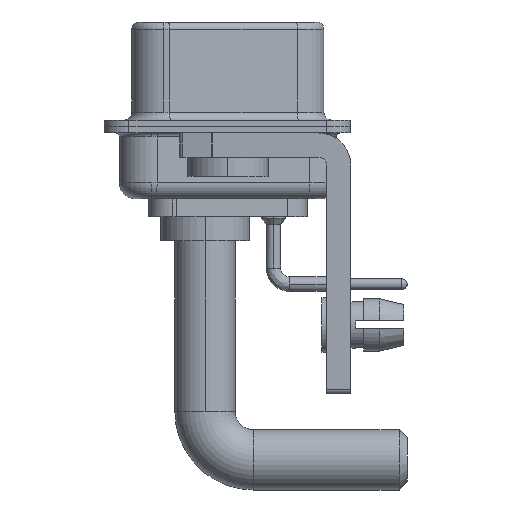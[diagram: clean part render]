
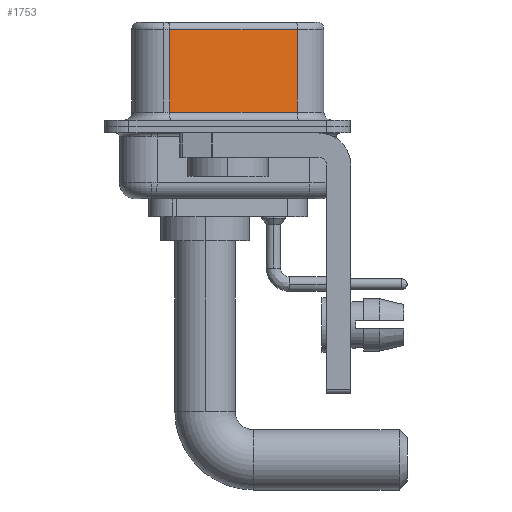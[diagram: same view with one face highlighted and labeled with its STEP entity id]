
A CAD part, left-side view. The second image highlights one B-rep face of the part: STEP entity #1753.
In plain terms, the highlighted planar face has unit normal (-0.985, -0.174, 0).
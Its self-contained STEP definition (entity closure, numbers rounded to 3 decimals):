
#435 = ORIENTED_EDGE ( 'NONE', *, *, #20019, .F. ) ;
#1753 = ADVANCED_FACE ( 'NONE', ( #7805 ), #26014, .F. ) ;
#2427 = LINE ( 'NONE', #4057, #3709 ) ;
#3034 = EDGE_CURVE ( 'NONE', #8544, #25024, #25427, .T. ) ;
#3056 = CARTESIAN_POINT ( 'NONE',  ( 5.132, -4.322, 6.02 ) ) ;
#3384 = CARTESIAN_POINT ( 'NONE',  ( 5.132, -4.322, 6.52 ) ) ;
#3709 = VECTOR ( 'NONE', #14762, 1000. ) ;
#4057 = CARTESIAN_POINT ( 'NONE',  ( 5.132, -4.322, 0.9 ) ) ;
#5459 = DIRECTION ( 'NONE',  ( -0.174, 0.985, 0. ) ) ;
#5599 = DIRECTION ( 'NONE',  ( 0., 0., -1. ) ) ;
#6811 = AXIS2_PLACEMENT_3D ( 'NONE', #3384, #19721, #7542 ) ;
#7191 = EDGE_LOOP ( 'NONE', ( #435, #9378, #7311, #12192 ) ) ;
#7311 = ORIENTED_EDGE ( 'NONE', *, *, #17206, .T. ) ;
#7542 = DIRECTION ( 'NONE',  ( -0.174, 0.985, 0. ) ) ;
#7805 = FACE_OUTER_BOUND ( 'NONE', #7191, .T. ) ;
#8544 = VERTEX_POINT ( 'NONE', #24185 ) ;
#9378 = ORIENTED_EDGE ( 'NONE', *, *, #3034, .T. ) ;
#12192 = ORIENTED_EDGE ( 'NONE', *, *, #13444, .T. ) ;
#13444 = EDGE_CURVE ( 'NONE', #19548, #16206, #2427, .T. ) ;
#14762 = DIRECTION ( 'NONE',  ( 0.174, -0.985, 0. ) ) ;
#15463 = VECTOR ( 'NONE', #21541, 1000. ) ;
#16206 = VERTEX_POINT ( 'NONE', #16583 ) ;
#16583 = CARTESIAN_POINT ( 'NONE',  ( 5.132, -4.322, 0.9 ) ) ;
#16731 = VECTOR ( 'NONE', #5459, 1000. ) ;
#17206 = EDGE_CURVE ( 'NONE', #25024, #19548, #21676, .T. ) ;
#17392 = CARTESIAN_POINT ( 'NONE',  ( 5.132, -4.322, 6.52 ) ) ;
#17436 = CARTESIAN_POINT ( 'NONE',  ( 3.73, 3.628, 6.02 ) ) ;
#19548 = VERTEX_POINT ( 'NONE', #19554 ) ;
#19554 = CARTESIAN_POINT ( 'NONE',  ( 3.73, 3.628, 0.9 ) ) ;
#19721 = DIRECTION ( 'NONE',  ( 0.985, 0.174, 0. ) ) ;
#19935 = CARTESIAN_POINT ( 'NONE',  ( 3.73, 3.628, 6.52 ) ) ;
#20019 = EDGE_CURVE ( 'NONE', #8544, #16206, #23542, .T. ) ;
#21541 = DIRECTION ( 'NONE',  ( 0., 0., -1. ) ) ;
#21676 = LINE ( 'NONE', #19935, #22608 ) ;
#22608 = VECTOR ( 'NONE', #5599, 1000. ) ;
#23542 = LINE ( 'NONE', #17392, #15463 ) ;
#24185 = CARTESIAN_POINT ( 'NONE',  ( 5.132, -4.322, 6.02 ) ) ;
#25024 = VERTEX_POINT ( 'NONE', #17436 ) ;
#25427 = LINE ( 'NONE', #3056, #16731 ) ;
#26014 = PLANE ( 'NONE',  #6811 ) ;
